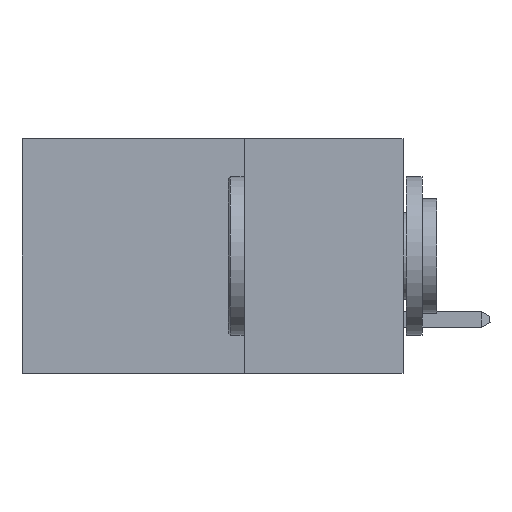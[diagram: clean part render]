
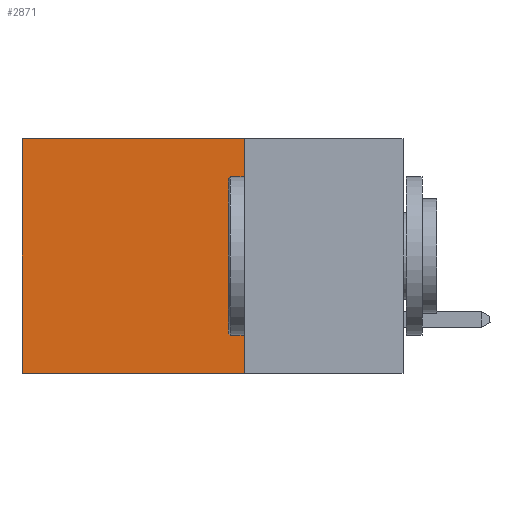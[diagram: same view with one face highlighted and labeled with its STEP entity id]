
A CAD part, left-side view. The second image highlights one B-rep face of the part: STEP entity #2871.
In plain terms, the highlighted planar face has unit normal (-1, 0, 0).
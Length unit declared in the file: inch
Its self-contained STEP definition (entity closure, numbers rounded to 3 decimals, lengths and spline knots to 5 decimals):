
#628 = VECTOR ( 'NONE', #41565, 39.37008 ) ;
#2871 = ADVANCED_FACE ( 'NONE', ( #11282 ), #12383, .F. ) ;
#4100 = DIRECTION ( 'NONE',  ( 0., 0., -1. ) ) ;
#4282 = CARTESIAN_POINT ( 'NONE',  ( 0.2875, 0.25, 0. ) ) ;
#6288 = CARTESIAN_POINT ( 'NONE',  ( 0.2875, 0.6, 0. ) ) ;
#6890 = ORIENTED_EDGE ( 'NONE', *, *, #22690, .T. ) ;
#11282 = FACE_OUTER_BOUND ( 'NONE', #21506, .T. ) ;
#12383 = PLANE ( 'NONE',  #44101 ) ;
#12971 = VERTEX_POINT ( 'NONE', #15770 ) ;
#15770 = CARTESIAN_POINT ( 'NONE',  ( 0.2875, 0.25, -0.37 ) ) ;
#17134 = LINE ( 'NONE', #28326, #36738 ) ;
#17625 = DIRECTION ( 'NONE',  ( 0., 1., 0. ) ) ;
#19055 = VERTEX_POINT ( 'NONE', #48465 ) ;
#19074 = LINE ( 'NONE', #37300, #37448 ) ;
#21506 = EDGE_LOOP ( 'NONE', ( #28551, #39194, #28376, #6890 ) ) ;
#22106 = LINE ( 'NONE', #6288, #628 ) ;
#22690 = EDGE_CURVE ( 'NONE', #30344, #41155, #17134, .T. ) ;
#23442 = CARTESIAN_POINT ( 'NONE',  ( 0.2875, 0.25, 0. ) ) ;
#24775 = CARTESIAN_POINT ( 'NONE',  ( 0.2875, 0.25, 0. ) ) ;
#28064 = CARTESIAN_POINT ( 'NONE',  ( 0.2875, 0.6, 0. ) ) ;
#28326 = CARTESIAN_POINT ( 'NONE',  ( 0.2875, 0.25, 0. ) ) ;
#28376 = ORIENTED_EDGE ( 'NONE', *, *, #34174, .F. ) ;
#28395 = LINE ( 'NONE', #23442, #42528 ) ;
#28551 = ORIENTED_EDGE ( 'NONE', *, *, #35932, .T. ) ;
#30344 = VERTEX_POINT ( 'NONE', #24775 ) ;
#34174 = EDGE_CURVE ( 'NONE', #30344, #12971, #28395, .T. ) ;
#35690 = EDGE_CURVE ( 'NONE', #12971, #19055, #19074, .T. ) ;
#35818 = DIRECTION ( 'NONE',  ( 1., 0., 0. ) ) ;
#35932 = EDGE_CURVE ( 'NONE', #41155, #19055, #22106, .T. ) ;
#36738 = VECTOR ( 'NONE', #48398, 39.37008 ) ;
#37300 = CARTESIAN_POINT ( 'NONE',  ( 0.2875, 0.25, -0.37 ) ) ;
#37448 = VECTOR ( 'NONE', #17625, 39.37008 ) ;
#39194 = ORIENTED_EDGE ( 'NONE', *, *, #35690, .F. ) ;
#41155 = VERTEX_POINT ( 'NONE', #28064 ) ;
#41565 = DIRECTION ( 'NONE',  ( 0., 0., -1. ) ) ;
#42528 = VECTOR ( 'NONE', #4100, 39.37008 ) ;
#43522 = DIRECTION ( 'NONE',  ( 0., 0., -1. ) ) ;
#44101 = AXIS2_PLACEMENT_3D ( 'NONE', #4282, #35818, #43522 ) ;
#48398 = DIRECTION ( 'NONE',  ( 0., 1., 0. ) ) ;
#48465 = CARTESIAN_POINT ( 'NONE',  ( 0.2875, 0.6, -0.37 ) ) ;
